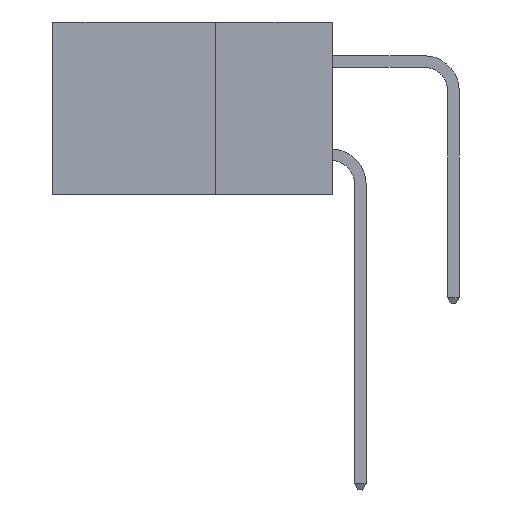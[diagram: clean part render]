
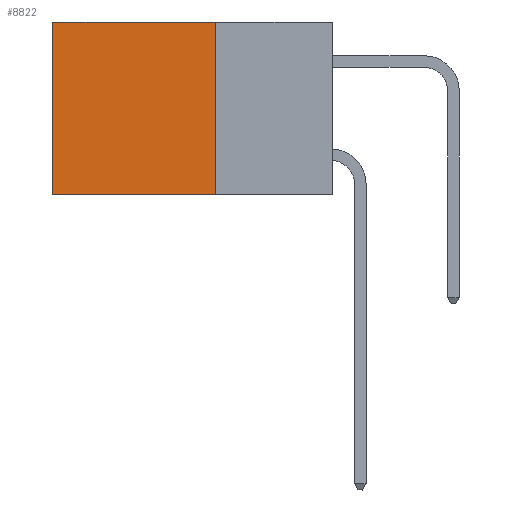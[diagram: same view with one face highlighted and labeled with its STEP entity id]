
A CAD part, left-side view. The second image highlights one B-rep face of the part: STEP entity #8822.
In plain terms, the highlighted planar face has unit normal (-1, 0, 0).
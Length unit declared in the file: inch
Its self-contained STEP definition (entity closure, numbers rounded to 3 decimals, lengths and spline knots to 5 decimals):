
#253 = CARTESIAN_POINT ( 'NONE',  ( 0.298, 0.25, 0. ) ) ;
#837 = EDGE_CURVE ( 'NONE', #12081, #2574, #15670, .T. ) ;
#1085 = VERTEX_POINT ( 'NONE', #15483 ) ;
#1112 = ORIENTED_EDGE ( 'NONE', *, *, #4388, .T. ) ;
#1544 = ORIENTED_EDGE ( 'NONE', *, *, #8328, .F. ) ;
#2574 = VERTEX_POINT ( 'NONE', #16931 ) ;
#2671 = VECTOR ( 'NONE', #4189, 39.37008 ) ;
#3080 = DIRECTION ( 'NONE',  ( 0., 0., -1. ) ) ;
#3086 = EDGE_CURVE ( 'NONE', #12081, #1085, #3528, .T. ) ;
#3528 = LINE ( 'NONE', #9083, #2671 ) ;
#4189 = DIRECTION ( 'NONE',  ( 0., 0., -1. ) ) ;
#4388 = EDGE_CURVE ( 'NONE', #2574, #8434, #14908, .T. ) ;
#4977 = CARTESIAN_POINT ( 'NONE',  ( 0.298, 0.6, -0.37 ) ) ;
#5059 = VECTOR ( 'NONE', #8655, 39.37008 ) ;
#5534 = ORIENTED_EDGE ( 'NONE', *, *, #837, .T. ) ;
#5901 = EDGE_LOOP ( 'NONE', ( #1112, #1544, #15278, #5534 ) ) ;
#7363 = CARTESIAN_POINT ( 'NONE',  ( 0.298, 0.25, -0.37 ) ) ;
#7807 = VECTOR ( 'NONE', #13200, 39.37008 ) ;
#8153 = CARTESIAN_POINT ( 'NONE',  ( 0.298, 0.25, 0. ) ) ;
#8328 = EDGE_CURVE ( 'NONE', #1085, #8434, #15612, .T. ) ;
#8434 = VERTEX_POINT ( 'NONE', #4977 ) ;
#8655 = DIRECTION ( 'NONE',  ( 0., 1., 0. ) ) ;
#8822 = ADVANCED_FACE ( 'NONE', ( #11621 ), #9579, .F. ) ;
#9083 = CARTESIAN_POINT ( 'NONE',  ( 0.298, 0.25, 0. ) ) ;
#9579 = PLANE ( 'NONE',  #13970 ) ;
#10869 = DIRECTION ( 'NONE',  ( 1., 0., 0. ) ) ;
#11621 = FACE_OUTER_BOUND ( 'NONE', #5901, .T. ) ;
#12081 = VERTEX_POINT ( 'NONE', #8153 ) ;
#12312 = VECTOR ( 'NONE', #15335, 39.37008 ) ;
#13200 = DIRECTION ( 'NONE',  ( 0., 0., -1. ) ) ;
#13367 = CARTESIAN_POINT ( 'NONE',  ( 0.298, 0.6, 0. ) ) ;
#13970 = AXIS2_PLACEMENT_3D ( 'NONE', #253, #10869, #3080 ) ;
#14908 = LINE ( 'NONE', #13367, #7807 ) ;
#15278 = ORIENTED_EDGE ( 'NONE', *, *, #3086, .F. ) ;
#15284 = CARTESIAN_POINT ( 'NONE',  ( 0.298, 0.25, 0. ) ) ;
#15335 = DIRECTION ( 'NONE',  ( 0., 1., 0. ) ) ;
#15483 = CARTESIAN_POINT ( 'NONE',  ( 0.298, 0.25, -0.37 ) ) ;
#15612 = LINE ( 'NONE', #7363, #5059 ) ;
#15670 = LINE ( 'NONE', #15284, #12312 ) ;
#16931 = CARTESIAN_POINT ( 'NONE',  ( 0.298, 0.6, 0. ) ) ;
